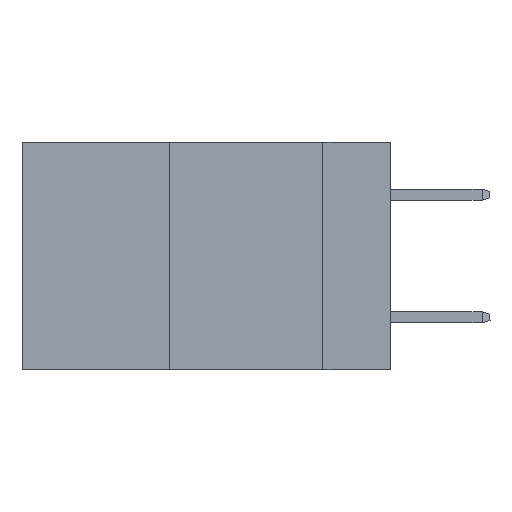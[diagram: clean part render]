
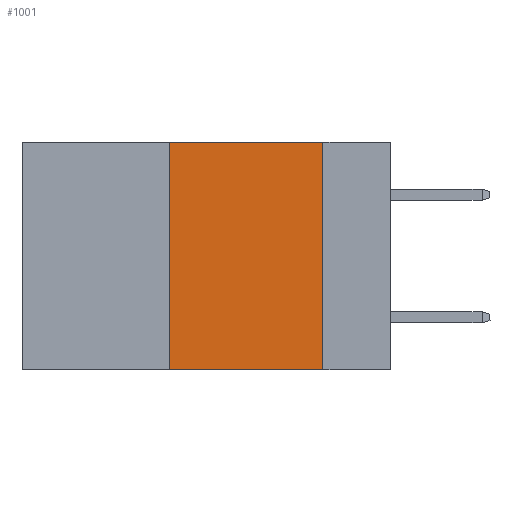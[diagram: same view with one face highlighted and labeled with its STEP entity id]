
A CAD part, left-side view. The second image highlights one B-rep face of the part: STEP entity #1001.
In plain terms, the highlighted planar face has unit normal (-1, 0, 0).
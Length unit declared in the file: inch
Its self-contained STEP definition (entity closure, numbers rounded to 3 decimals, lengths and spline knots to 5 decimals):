
#19 = EDGE_LOOP ( 'NONE', ( #4281, #206, #8752, #10773 ) ) ;
#206 = ORIENTED_EDGE ( 'NONE', *, *, #798, .F. ) ;
#408 = DIRECTION ( 'NONE',  ( 0., -1., 0. ) ) ;
#475 = VERTEX_POINT ( 'NONE', #4033 ) ;
#798 = EDGE_CURVE ( 'NONE', #2314, #2610, #5857, .T. ) ;
#873 = VECTOR ( 'NONE', #6732, 39.37008 ) ;
#1001 = ADVANCED_FACE ( 'NONE', ( #4466 ), #8062, .F. ) ;
#1111 = CARTESIAN_POINT ( 'NONE',  ( 0., 0.36, -0.37 ) ) ;
#1992 = DIRECTION ( 'NONE',  ( 0., 0., -1. ) ) ;
#2098 = CARTESIAN_POINT ( 'NONE',  ( 0., 0.6, 0. ) ) ;
#2192 = CARTESIAN_POINT ( 'NONE',  ( 0., 0.36, 0. ) ) ;
#2215 = AXIS2_PLACEMENT_3D ( 'NONE', #8141, #4600, #1992 ) ;
#2314 = VERTEX_POINT ( 'NONE', #2192 ) ;
#2610 = VERTEX_POINT ( 'NONE', #8732 ) ;
#3014 = VERTEX_POINT ( 'NONE', #1111 ) ;
#3528 = LINE ( 'NONE', #3816, #4481 ) ;
#3816 = CARTESIAN_POINT ( 'NONE',  ( 0., 0.11, 0. ) ) ;
#4029 = VECTOR ( 'NONE', #408, 39.37008 ) ;
#4033 = CARTESIAN_POINT ( 'NONE',  ( 0., 0.11, -0.37 ) ) ;
#4281 = ORIENTED_EDGE ( 'NONE', *, *, #10013, .F. ) ;
#4466 = FACE_OUTER_BOUND ( 'NONE', #19, .T. ) ;
#4481 = VECTOR ( 'NONE', #10981, 39.37008 ) ;
#4600 = DIRECTION ( 'NONE',  ( 1., 0., 0. ) ) ;
#4814 = LINE ( 'NONE', #8354, #4029 ) ;
#5358 = VECTOR ( 'NONE', #10115, 39.37008 ) ;
#5857 = LINE ( 'NONE', #2098, #5358 ) ;
#6732 = DIRECTION ( 'NONE',  ( 0., 0., 1. ) ) ;
#6852 = CARTESIAN_POINT ( 'NONE',  ( 0., 0.36, 0. ) ) ;
#6853 = EDGE_CURVE ( 'NONE', #3014, #475, #4814, .T. ) ;
#7542 = LINE ( 'NONE', #6852, #873 ) ;
#8062 = PLANE ( 'NONE',  #2215 ) ;
#8080 = EDGE_CURVE ( 'NONE', #3014, #2314, #7542, .T. ) ;
#8141 = CARTESIAN_POINT ( 'NONE',  ( 0., 0.6, 0. ) ) ;
#8354 = CARTESIAN_POINT ( 'NONE',  ( 0., 0.6, -0.37 ) ) ;
#8732 = CARTESIAN_POINT ( 'NONE',  ( 0., 0.11, 0. ) ) ;
#8752 = ORIENTED_EDGE ( 'NONE', *, *, #8080, .F. ) ;
#10013 = EDGE_CURVE ( 'NONE', #2610, #475, #3528, .T. ) ;
#10115 = DIRECTION ( 'NONE',  ( 0., -1., 0. ) ) ;
#10773 = ORIENTED_EDGE ( 'NONE', *, *, #6853, .T. ) ;
#10981 = DIRECTION ( 'NONE',  ( 0., 0., -1. ) ) ;
